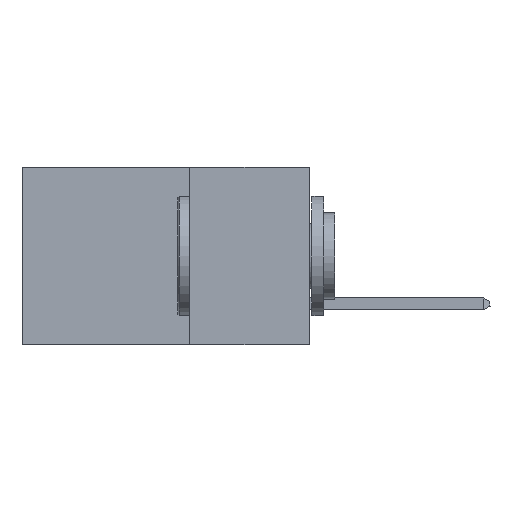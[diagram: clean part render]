
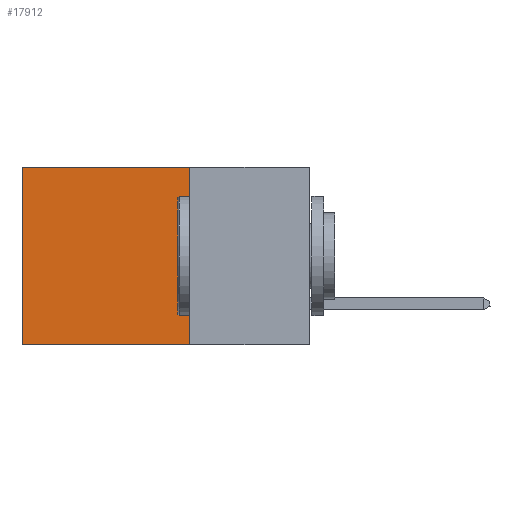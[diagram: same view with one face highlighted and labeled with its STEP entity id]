
A CAD part, left-side view. The second image highlights one B-rep face of the part: STEP entity #17912.
In plain terms, the highlighted planar face has unit normal (-1, 0, 0).
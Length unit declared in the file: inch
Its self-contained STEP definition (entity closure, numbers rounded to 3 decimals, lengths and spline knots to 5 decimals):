
#470 = EDGE_CURVE ( 'NONE', #2278, #31100, #29364, .T. ) ;
#2278 = VERTEX_POINT ( 'NONE', #10169 ) ;
#3388 = ORIENTED_EDGE ( 'NONE', *, *, #470, .T. ) ;
#3547 = ORIENTED_EDGE ( 'NONE', *, *, #34976, .F. ) ;
#3798 = DIRECTION ( 'NONE',  ( 0., 0., -1. ) ) ;
#5236 = CARTESIAN_POINT ( 'NONE',  ( 0.2875, 0.25, 0. ) ) ;
#5977 = CARTESIAN_POINT ( 'NONE',  ( 0.2875, 0.6, 0. ) ) ;
#9440 = DIRECTION ( 'NONE',  ( 0., 1., 0. ) ) ;
#10169 = CARTESIAN_POINT ( 'NONE',  ( 0.2875, 0.25, 0. ) ) ;
#11795 = VECTOR ( 'NONE', #9440, 39.37008 ) ;
#12812 = CARTESIAN_POINT ( 'NONE',  ( 0.2875, 0.25, 0. ) ) ;
#13011 = LINE ( 'NONE', #47308, #11795 ) ;
#14950 = EDGE_CURVE ( 'NONE', #31100, #33345, #41471, .T. ) ;
#15315 = VERTEX_POINT ( 'NONE', #17554 ) ;
#17554 = CARTESIAN_POINT ( 'NONE',  ( 0.2875, 0.25, -0.37 ) ) ;
#17912 = ADVANCED_FACE ( 'NONE', ( #26769 ), #23195, .F. ) ;
#18988 = CARTESIAN_POINT ( 'NONE',  ( 0.2875, 0.25, 0. ) ) ;
#23128 = DIRECTION ( 'NONE',  ( 0., 0., -1. ) ) ;
#23195 = PLANE ( 'NONE',  #24325 ) ;
#24325 = AXIS2_PLACEMENT_3D ( 'NONE', #18988, #30814, #3798 ) ;
#25224 = EDGE_LOOP ( 'NONE', ( #31413, #33610, #3547, #3388 ) ) ;
#26261 = CARTESIAN_POINT ( 'NONE',  ( 0.2875, 0.6, -0.37 ) ) ;
#26769 = FACE_OUTER_BOUND ( 'NONE', #25224, .T. ) ;
#26944 = VECTOR ( 'NONE', #35904, 39.37008 ) ;
#29364 = LINE ( 'NONE', #5236, #26944 ) ;
#30814 = DIRECTION ( 'NONE',  ( 1., 0., 0. ) ) ;
#31100 = VERTEX_POINT ( 'NONE', #5977 ) ;
#31413 = ORIENTED_EDGE ( 'NONE', *, *, #14950, .T. ) ;
#33345 = VERTEX_POINT ( 'NONE', #26261 ) ;
#33610 = ORIENTED_EDGE ( 'NONE', *, *, #40633, .F. ) ;
#34976 = EDGE_CURVE ( 'NONE', #2278, #15315, #39367, .T. ) ;
#35904 = DIRECTION ( 'NONE',  ( 0., 1., 0. ) ) ;
#38723 = CARTESIAN_POINT ( 'NONE',  ( 0.2875, 0.6, 0. ) ) ;
#39277 = DIRECTION ( 'NONE',  ( 0., 0., -1. ) ) ;
#39367 = LINE ( 'NONE', #12812, #43543 ) ;
#40633 = EDGE_CURVE ( 'NONE', #15315, #33345, #13011, .T. ) ;
#41471 = LINE ( 'NONE', #38723, #43843 ) ;
#43543 = VECTOR ( 'NONE', #39277, 39.37008 ) ;
#43843 = VECTOR ( 'NONE', #23128, 39.37008 ) ;
#47308 = CARTESIAN_POINT ( 'NONE',  ( 0.2875, 0.25, -0.37 ) ) ;
